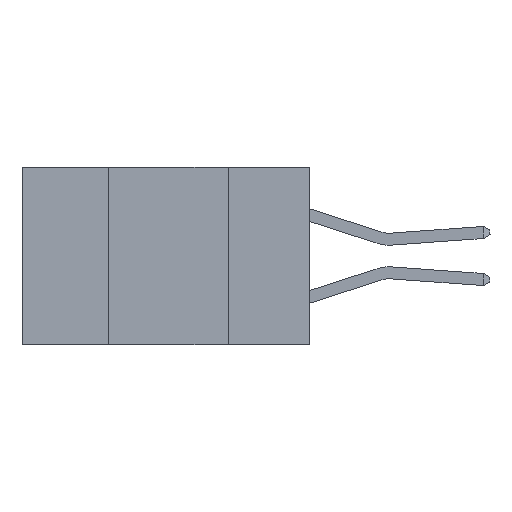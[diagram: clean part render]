
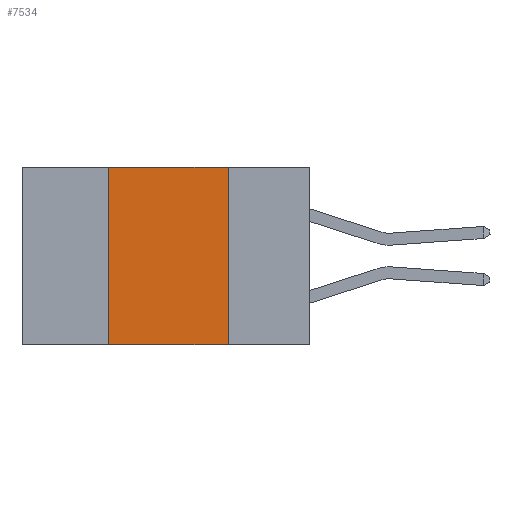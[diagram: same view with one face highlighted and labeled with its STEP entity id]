
A CAD part, left-side view. The second image highlights one B-rep face of the part: STEP entity #7534.
In plain terms, the highlighted planar face has unit normal (-1, 0, 0).
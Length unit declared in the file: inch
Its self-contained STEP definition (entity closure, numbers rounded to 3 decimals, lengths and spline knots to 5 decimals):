
#288 = VECTOR ( 'NONE', #10338, 39.37008 ) ;
#629 = EDGE_CURVE ( 'NONE', #4343, #15563, #6386, .T. ) ;
#1111 = CARTESIAN_POINT ( 'NONE',  ( 0., 0.6, 0. ) ) ;
#1442 = CARTESIAN_POINT ( 'NONE',  ( 0., 0.17, 0. ) ) ;
#1893 = DIRECTION ( 'NONE',  ( 0., -1., 0. ) ) ;
#2225 = ORIENTED_EDGE ( 'NONE', *, *, #11692, .F. ) ;
#2323 = CARTESIAN_POINT ( 'NONE',  ( 0., 0.6, -0.37 ) ) ;
#3496 = VERTEX_POINT ( 'NONE', #1442 ) ;
#3768 = CARTESIAN_POINT ( 'NONE',  ( 0., 0.42, 0. ) ) ;
#3974 = CARTESIAN_POINT ( 'NONE',  ( 0., 0.17, -0.37 ) ) ;
#4343 = VERTEX_POINT ( 'NONE', #13995 ) ;
#4585 = VERTEX_POINT ( 'NONE', #3768 ) ;
#4759 = CARTESIAN_POINT ( 'NONE',  ( 0., 0.6, 0. ) ) ;
#5541 = ORIENTED_EDGE ( 'NONE', *, *, #7559, .F. ) ;
#6386 = LINE ( 'NONE', #2323, #288 ) ;
#7114 = VECTOR ( 'NONE', #17960, 39.37008 ) ;
#7534 = ADVANCED_FACE ( 'NONE', ( #17945 ), #12511, .F. ) ;
#7559 = EDGE_CURVE ( 'NONE', #4343, #4585, #13904, .T. ) ;
#7921 = DIRECTION ( 'NONE',  ( 0., 0., -1. ) ) ;
#8068 = AXIS2_PLACEMENT_3D ( 'NONE', #1111, #12432, #7921 ) ;
#8205 = DIRECTION ( 'NONE',  ( 0., 0., 1. ) ) ;
#8320 = EDGE_CURVE ( 'NONE', #4585, #3496, #13037, .T. ) ;
#9839 = ORIENTED_EDGE ( 'NONE', *, *, #629, .T. ) ;
#10338 = DIRECTION ( 'NONE',  ( 0., -1., 0. ) ) ;
#11005 = VECTOR ( 'NONE', #8205, 39.37008 ) ;
#11692 = EDGE_CURVE ( 'NONE', #3496, #15563, #12619, .T. ) ;
#12337 = CARTESIAN_POINT ( 'NONE',  ( 0., 0.42, -0.37 ) ) ;
#12432 = DIRECTION ( 'NONE',  ( 1., 0., 0. ) ) ;
#12511 = PLANE ( 'NONE',  #8068 ) ;
#12619 = LINE ( 'NONE', #3974, #7114 ) ;
#13037 = LINE ( 'NONE', #4759, #15328 ) ;
#13904 = LINE ( 'NONE', #12337, #11005 ) ;
#13995 = CARTESIAN_POINT ( 'NONE',  ( 0., 0.42, -0.37 ) ) ;
#14379 = CARTESIAN_POINT ( 'NONE',  ( 0., 0.17, -0.37 ) ) ;
#15122 = ORIENTED_EDGE ( 'NONE', *, *, #8320, .F. ) ;
#15328 = VECTOR ( 'NONE', #1893, 39.37008 ) ;
#15377 = EDGE_LOOP ( 'NONE', ( #2225, #15122, #5541, #9839 ) ) ;
#15563 = VERTEX_POINT ( 'NONE', #14379 ) ;
#17945 = FACE_OUTER_BOUND ( 'NONE', #15377, .T. ) ;
#17960 = DIRECTION ( 'NONE',  ( 0., 0., -1. ) ) ;
